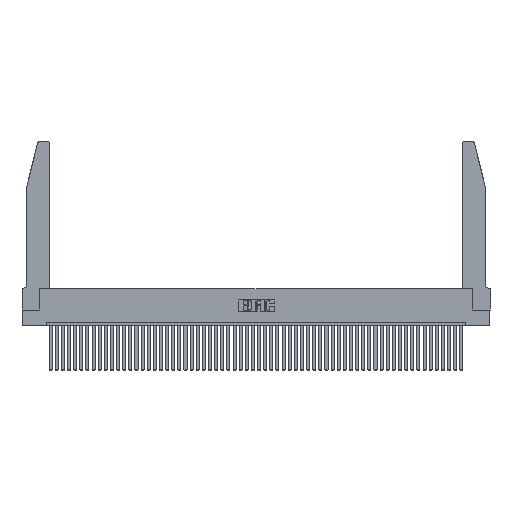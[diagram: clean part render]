
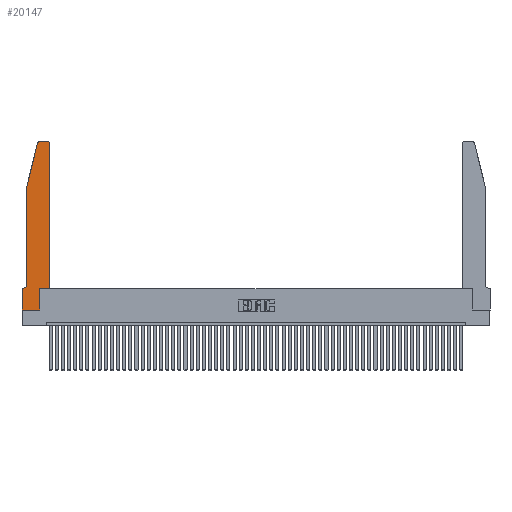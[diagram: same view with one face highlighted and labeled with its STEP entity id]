
A CAD part, top view. The second image highlights one B-rep face of the part: STEP entity #20147.
In plain terms, the highlighted planar face has unit normal (0, 0, 1).
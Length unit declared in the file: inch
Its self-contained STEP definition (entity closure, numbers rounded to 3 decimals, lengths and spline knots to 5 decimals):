
#22 = CARTESIAN_POINT ( 'NONE',  ( 0.0055, 0.35, 0.37 ) ) ;
#378 = VECTOR ( 'NONE', #38342, 39.37008 ) ;
#893 = CARTESIAN_POINT ( 'NONE',  ( 0.4205, 2.72, 0.37 ) ) ;
#1243 = CARTESIAN_POINT ( 'NONE',  ( 0.0755, 2., 0.37 ) ) ;
#2559 = VECTOR ( 'NONE', #38401, 39.37008 ) ;
#3823 = LINE ( 'NONE', #6657, #2559 ) ;
#5122 = DIRECTION ( 'NONE',  ( -1., 0., 0. ) ) ;
#5293 = VERTEX_POINT ( 'NONE', #47733 ) ;
#5441 = ORIENTED_EDGE ( 'NONE', *, *, #36496, .T. ) ;
#5915 = CARTESIAN_POINT ( 'NONE',  ( 0.284, 2.72, 0.37 ) ) ;
#6300 = ORIENTED_EDGE ( 'NONE', *, *, #6810, .T. ) ;
#6657 = CARTESIAN_POINT ( 'NONE',  ( 0.2865, 0.35, 0.37 ) ) ;
#6774 = VECTOR ( 'NONE', #23211, 39.37008 ) ;
#6808 = CARTESIAN_POINT ( 'NONE',  ( 0.4205, 2.75, 0.37 ) ) ;
#6810 = EDGE_CURVE ( 'NONE', #47627, #14363, #47224, .T. ) ;
#6822 = CARTESIAN_POINT ( 'NONE',  ( 0., 0.35, 0.37 ) ) ;
#7466 = VERTEX_POINT ( 'NONE', #6808 ) ;
#9186 = DIRECTION ( 'NONE',  ( 0., 0., 1. ) ) ;
#9929 = CARTESIAN_POINT ( 'NONE',  ( 0.4505, 0.35, 0.37 ) ) ;
#10919 = VERTEX_POINT ( 'NONE', #21364 ) ;
#11226 = VERTEX_POINT ( 'NONE', #35425 ) ;
#11709 = ORIENTED_EDGE ( 'NONE', *, *, #45363, .T. ) ;
#12170 = VERTEX_POINT ( 'NONE', #12223 ) ;
#12223 = CARTESIAN_POINT ( 'NONE',  ( 0.0755, 2., 0.37 ) ) ;
#12433 = LINE ( 'NONE', #1243, #31386 ) ;
#12777 = ORIENTED_EDGE ( 'NONE', *, *, #31917, .T. ) ;
#13026 = LINE ( 'NONE', #9929, #378 ) ;
#14116 = LINE ( 'NONE', #16148, #30917 ) ;
#14363 = VERTEX_POINT ( 'NONE', #22 ) ;
#15473 = EDGE_CURVE ( 'NONE', #44574, #7466, #30579, .T. ) ;
#16148 = CARTESIAN_POINT ( 'NONE',  ( 0.0755, 0.35, 0.37 ) ) ;
#16964 = DIRECTION ( 'NONE',  ( 1., 0., 0. ) ) ;
#17568 = DIRECTION ( 'NONE',  ( 1., 0., 0. ) ) ;
#18273 = CIRCLE ( 'NONE', #48872, 0.03 ) ;
#18739 = VERTEX_POINT ( 'NONE', #42407 ) ;
#18782 = LINE ( 'NONE', #31327, #6774 ) ;
#20147 = ADVANCED_FACE ( 'NONE', ( #44580 ), #42811, .T. ) ;
#20491 = AXIS2_PLACEMENT_3D ( 'NONE', #50561, #33851, #20978 ) ;
#20978 = DIRECTION ( 'NONE',  ( -1., 0., 0. ) ) ;
#21364 = CARTESIAN_POINT ( 'NONE',  ( 0., 0., 0.37 ) ) ;
#22393 = CARTESIAN_POINT ( 'NONE',  ( 0.0755, 2., 0.37 ) ) ;
#22421 = LINE ( 'NONE', #36610, #26235 ) ;
#22547 = CARTESIAN_POINT ( 'NONE',  ( 0.0755, 0.42, 0.37 ) ) ;
#23211 = DIRECTION ( 'NONE',  ( 1., 0., 0. ) ) ;
#23482 = VECTOR ( 'NONE', #5122, 39.37008 ) ;
#24279 = DIRECTION ( 'NONE',  ( 0., -1., 0. ) ) ;
#24294 = CARTESIAN_POINT ( 'NONE',  ( 0.4505, 0.35, 0.37 ) ) ;
#25549 = CARTESIAN_POINT ( 'NONE',  ( 0.4505, 0.35, 0.37 ) ) ;
#26019 = LINE ( 'NONE', #41132, #23482 ) ;
#26235 = VECTOR ( 'NONE', #24279, 39.37008 ) ;
#27857 = ORIENTED_EDGE ( 'NONE', *, *, #31462, .T. ) ;
#28540 = CARTESIAN_POINT ( 'NONE',  ( 0.4505, 2.72, 0.37 ) ) ;
#29118 = LINE ( 'NONE', #22393, #48087 ) ;
#30470 = DIRECTION ( 'NONE',  ( 0., -1., 0. ) ) ;
#30579 = CIRCLE ( 'NONE', #33202, 0.03 ) ;
#30737 = EDGE_CURVE ( 'NONE', #5293, #12170, #12433, .T. ) ;
#30917 = VECTOR ( 'NONE', #31859, 39.37008 ) ;
#31327 = CARTESIAN_POINT ( 'NONE',  ( 0., 0., 0.37 ) ) ;
#31386 = VECTOR ( 'NONE', #33006, 39.37008 ) ;
#31462 = EDGE_CURVE ( 'NONE', #12170, #47627, #29118, .T. ) ;
#31859 = DIRECTION ( 'NONE',  ( -1., 0., 0. ) ) ;
#31879 = CARTESIAN_POINT ( 'NONE',  ( 0.284, 2.75, 0.37 ) ) ;
#31917 = EDGE_CURVE ( 'NONE', #40269, #5293, #18273, .T. ) ;
#33006 = DIRECTION ( 'NONE',  ( -0.239, -0.971, 0. ) ) ;
#33202 = AXIS2_PLACEMENT_3D ( 'NONE', #893, #9186, #16964 ) ;
#33851 = DIRECTION ( 'NONE',  ( 0., 0., -1. ) ) ;
#35160 = ORIENTED_EDGE ( 'NONE', *, *, #46041, .T. ) ;
#35221 = ORIENTED_EDGE ( 'NONE', *, *, #50348, .T. ) ;
#35425 = CARTESIAN_POINT ( 'NONE',  ( 0.2865, 0., 0.37 ) ) ;
#35471 = LINE ( 'NONE', #25549, #38007 ) ;
#36496 = EDGE_CURVE ( 'NONE', #40753, #52096, #35471, .T. ) ;
#36610 = CARTESIAN_POINT ( 'NONE',  ( 0., 0., 0.37 ) ) ;
#37332 = ORIENTED_EDGE ( 'NONE', *, *, #50721, .T. ) ;
#38007 = VECTOR ( 'NONE', #41570, 39.37008 ) ;
#38072 = AXIS2_PLACEMENT_3D ( 'NONE', #6822, #51052, #47025 ) ;
#38342 = DIRECTION ( 'NONE',  ( 0., 1., 0. ) ) ;
#38401 = DIRECTION ( 'NONE',  ( 0., 1., 0. ) ) ;
#39224 = ORIENTED_EDGE ( 'NONE', *, *, #30737, .T. ) ;
#40109 = CARTESIAN_POINT ( 'NONE',  ( 0.2865, 0.35, 0.37 ) ) ;
#40220 = ORIENTED_EDGE ( 'NONE', *, *, #49706, .T. ) ;
#40269 = VERTEX_POINT ( 'NONE', #31879 ) ;
#40753 = VERTEX_POINT ( 'NONE', #40109 ) ;
#41132 = CARTESIAN_POINT ( 'NONE',  ( 0.2605, 2.75, 0.37 ) ) ;
#41570 = DIRECTION ( 'NONE',  ( 1., 0., 0. ) ) ;
#42407 = CARTESIAN_POINT ( 'NONE',  ( 0., 0.35, 0.37 ) ) ;
#42811 = PLANE ( 'NONE',  #38072 ) ;
#44574 = VERTEX_POINT ( 'NONE', #28540 ) ;
#44580 = FACE_OUTER_BOUND ( 'NONE', #49476, .T. ) ;
#44960 = EDGE_CURVE ( 'NONE', #10919, #11226, #18782, .T. ) ;
#45363 = EDGE_CURVE ( 'NONE', #52096, #44574, #13026, .T. ) ;
#45437 = DIRECTION ( 'NONE',  ( 0., 0., 1. ) ) ;
#46041 = EDGE_CURVE ( 'NONE', #18739, #10919, #22421, .T. ) ;
#47025 = DIRECTION ( 'NONE',  ( 1., 0., 0. ) ) ;
#47224 = CIRCLE ( 'NONE', #20491, 0.07 ) ;
#47627 = VERTEX_POINT ( 'NONE', #22547 ) ;
#47733 = CARTESIAN_POINT ( 'NONE',  ( 0.25487, 2.72718, 0.37 ) ) ;
#47863 = ORIENTED_EDGE ( 'NONE', *, *, #44960, .T. ) ;
#48087 = VECTOR ( 'NONE', #30470, 39.37008 ) ;
#48872 = AXIS2_PLACEMENT_3D ( 'NONE', #5915, #45437, #17568 ) ;
#49217 = ORIENTED_EDGE ( 'NONE', *, *, #15473, .T. ) ;
#49476 = EDGE_LOOP ( 'NONE', ( #40220, #12777, #39224, #27857, #6300, #37332, #35160, #47863, #35221, #5441, #11709, #49217 ) ) ;
#49706 = EDGE_CURVE ( 'NONE', #7466, #40269, #26019, .T. ) ;
#50348 = EDGE_CURVE ( 'NONE', #11226, #40753, #3823, .T. ) ;
#50561 = CARTESIAN_POINT ( 'NONE',  ( 0.0055, 0.42, 0.37 ) ) ;
#50721 = EDGE_CURVE ( 'NONE', #14363, #18739, #14116, .T. ) ;
#51052 = DIRECTION ( 'NONE',  ( 0., 0., 1. ) ) ;
#52096 = VERTEX_POINT ( 'NONE', #24294 ) ;
